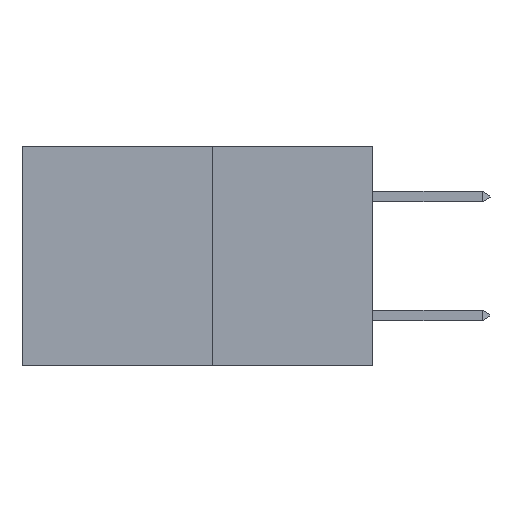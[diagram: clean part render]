
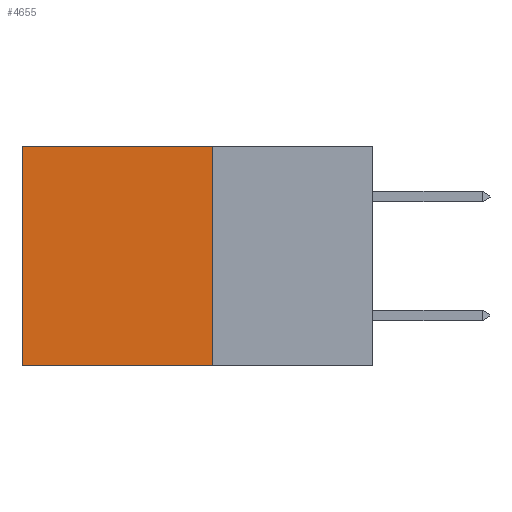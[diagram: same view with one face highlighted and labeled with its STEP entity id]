
A CAD part, left-side view. The second image highlights one B-rep face of the part: STEP entity #4655.
In plain terms, the highlighted planar face has unit normal (-1, 0, 0).
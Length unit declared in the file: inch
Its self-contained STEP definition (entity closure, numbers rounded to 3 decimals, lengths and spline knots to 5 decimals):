
#158 = LINE ( 'NONE', #12683, #12482 ) ;
#303 = LINE ( 'NONE', #7734, #15797 ) ;
#1266 = ORIENTED_EDGE ( 'NONE', *, *, #7877, .F. ) ;
#1437 = DIRECTION ( 'NONE',  ( 0., 1., 0. ) ) ;
#1444 = CARTESIAN_POINT ( 'NONE',  ( 0.277, 0.27, -0.37 ) ) ;
#2607 = EDGE_LOOP ( 'NONE', ( #9189, #1266, #15764, #7600 ) ) ;
#4655 = ADVANCED_FACE ( 'NONE', ( #5145 ), #11270, .F. ) ;
#5145 = FACE_OUTER_BOUND ( 'NONE', #2607, .T. ) ;
#5291 = VECTOR ( 'NONE', #13147, 39.37008 ) ;
#5473 = EDGE_CURVE ( 'NONE', #6892, #12434, #158, .T. ) ;
#5676 = CARTESIAN_POINT ( 'NONE',  ( 0.277, 0.59, 0. ) ) ;
#6053 = LINE ( 'NONE', #11936, #5291 ) ;
#6892 = VERTEX_POINT ( 'NONE', #7913 ) ;
#7256 = CARTESIAN_POINT ( 'NONE',  ( 0.277, 0.59, -0.37 ) ) ;
#7600 = ORIENTED_EDGE ( 'NONE', *, *, #13529, .T. ) ;
#7734 = CARTESIAN_POINT ( 'NONE',  ( 0.277, 0.59, -0.37 ) ) ;
#7877 = EDGE_CURVE ( 'NONE', #12434, #10029, #15272, .T. ) ;
#7913 = CARTESIAN_POINT ( 'NONE',  ( 0.277, 0.27, 0. ) ) ;
#8021 = EDGE_CURVE ( 'NONE', #12721, #10029, #303, .T. ) ;
#8488 = VECTOR ( 'NONE', #1437, 39.37008 ) ;
#9189 = ORIENTED_EDGE ( 'NONE', *, *, #8021, .T. ) ;
#10029 = VERTEX_POINT ( 'NONE', #7256 ) ;
#10528 = DIRECTION ( 'NONE',  ( 0., 0., -1. ) ) ;
#10620 = DIRECTION ( 'NONE',  ( 1., 0., 0. ) ) ;
#10759 = AXIS2_PLACEMENT_3D ( 'NONE', #11002, #10620, #10528 ) ;
#11002 = CARTESIAN_POINT ( 'NONE',  ( 0.277, 0.27, -0.37 ) ) ;
#11270 = PLANE ( 'NONE',  #10759 ) ;
#11936 = CARTESIAN_POINT ( 'NONE',  ( 0.277, 0.27, 0. ) ) ;
#12434 = VERTEX_POINT ( 'NONE', #1444 ) ;
#12482 = VECTOR ( 'NONE', #12592, 39.37008 ) ;
#12592 = DIRECTION ( 'NONE',  ( 0., 0., -1. ) ) ;
#12683 = CARTESIAN_POINT ( 'NONE',  ( 0.277, 0.27, -0.37 ) ) ;
#12721 = VERTEX_POINT ( 'NONE', #5676 ) ;
#13147 = DIRECTION ( 'NONE',  ( 0., 1., 0. ) ) ;
#13529 = EDGE_CURVE ( 'NONE', #6892, #12721, #6053, .T. ) ;
#14719 = CARTESIAN_POINT ( 'NONE',  ( 0.277, 0.27, -0.37 ) ) ;
#14979 = DIRECTION ( 'NONE',  ( 0., 0., -1. ) ) ;
#15272 = LINE ( 'NONE', #14719, #8488 ) ;
#15764 = ORIENTED_EDGE ( 'NONE', *, *, #5473, .F. ) ;
#15797 = VECTOR ( 'NONE', #14979, 39.37008 ) ;
